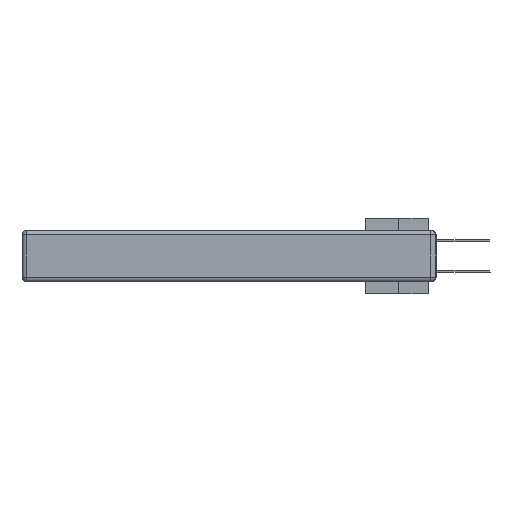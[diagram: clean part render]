
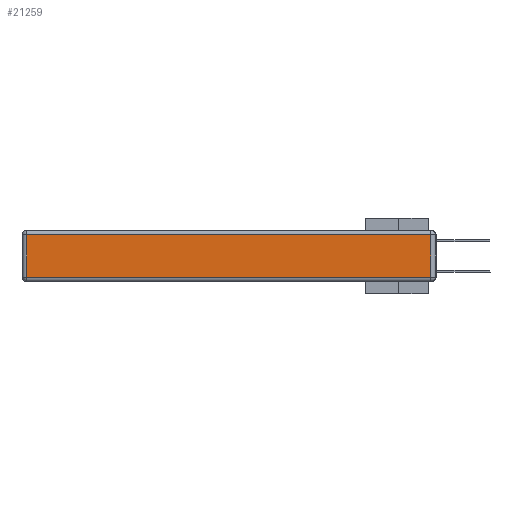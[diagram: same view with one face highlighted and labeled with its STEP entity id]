
A CAD part, left-side view. The second image highlights one B-rep face of the part: STEP entity #21259.
In plain terms, the highlighted planar face has unit normal (-1, 0, 0).
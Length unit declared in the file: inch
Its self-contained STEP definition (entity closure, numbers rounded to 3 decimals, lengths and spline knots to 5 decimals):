
#280 = EDGE_CURVE ( 'NONE', #29952, #13379, #2208, .T. ) ;
#577 = DIRECTION ( 'NONE',  ( 0., 1., 0. ) ) ;
#941 = CARTESIAN_POINT ( 'NONE',  ( 0., 2.72, -0.03 ) ) ;
#1530 = CARTESIAN_POINT ( 'NONE',  ( 0., 0., -0.343 ) ) ;
#1645 = DIRECTION ( 'NONE',  ( -1., 0., 0. ) ) ;
#1824 = VECTOR ( 'NONE', #19497, 39.37008 ) ;
#2208 = LINE ( 'NONE', #20718, #5285 ) ;
#3252 = VERTEX_POINT ( 'NONE', #941 ) ;
#5285 = VECTOR ( 'NONE', #29267, 39.37008 ) ;
#5542 = ORIENTED_EDGE ( 'NONE', *, *, #21439, .T. ) ;
#7094 = EDGE_LOOP ( 'NONE', ( #13670, #5542, #11548, #20056 ) ) ;
#11548 = ORIENTED_EDGE ( 'NONE', *, *, #25212, .T. ) ;
#12142 = CARTESIAN_POINT ( 'NONE',  ( 0., 2.75, -0.03 ) ) ;
#13379 = VERTEX_POINT ( 'NONE', #30111 ) ;
#13670 = ORIENTED_EDGE ( 'NONE', *, *, #280, .T. ) ;
#19497 = DIRECTION ( 'NONE',  ( 0., 0., -1. ) ) ;
#19582 = EDGE_CURVE ( 'NONE', #3252, #29952, #28948, .T. ) ;
#20056 = ORIENTED_EDGE ( 'NONE', *, *, #19582, .T. ) ;
#20718 = CARTESIAN_POINT ( 'NONE',  ( 0., 0., -0.313 ) ) ;
#21259 = ADVANCED_FACE ( 'NONE', ( #33603 ), #23673, .T. ) ;
#21439 = EDGE_CURVE ( 'NONE', #13379, #34048, #22278, .T. ) ;
#22278 = LINE ( 'NONE', #32475, #34052 ) ;
#23490 = CARTESIAN_POINT ( 'NONE',  ( 0., 0.03, -0.03 ) ) ;
#23673 = PLANE ( 'NONE',  #34030 ) ;
#25212 = EDGE_CURVE ( 'NONE', #34048, #3252, #28531, .T. ) ;
#27711 = CARTESIAN_POINT ( 'NONE',  ( 0., 2.72, -0.343 ) ) ;
#28531 = LINE ( 'NONE', #12142, #34198 ) ;
#28948 = LINE ( 'NONE', #27711, #1824 ) ;
#29267 = DIRECTION ( 'NONE',  ( 0., -1., 0. ) ) ;
#29841 = CARTESIAN_POINT ( 'NONE',  ( 0., 2.72, -0.313 ) ) ;
#29952 = VERTEX_POINT ( 'NONE', #29841 ) ;
#30111 = CARTESIAN_POINT ( 'NONE',  ( 0., 0.03, -0.313 ) ) ;
#32222 = DIRECTION ( 'NONE',  ( 0., 0., 1. ) ) ;
#32475 = CARTESIAN_POINT ( 'NONE',  ( 0., 0.03, -0.343 ) ) ;
#33603 = FACE_OUTER_BOUND ( 'NONE', #7094, .T. ) ;
#34030 = AXIS2_PLACEMENT_3D ( 'NONE', #1530, #1645, #32222 ) ;
#34048 = VERTEX_POINT ( 'NONE', #23490 ) ;
#34052 = VECTOR ( 'NONE', #35781, 39.37008 ) ;
#34198 = VECTOR ( 'NONE', #577, 39.37008 ) ;
#35781 = DIRECTION ( 'NONE',  ( 0., 0., 1. ) ) ;
